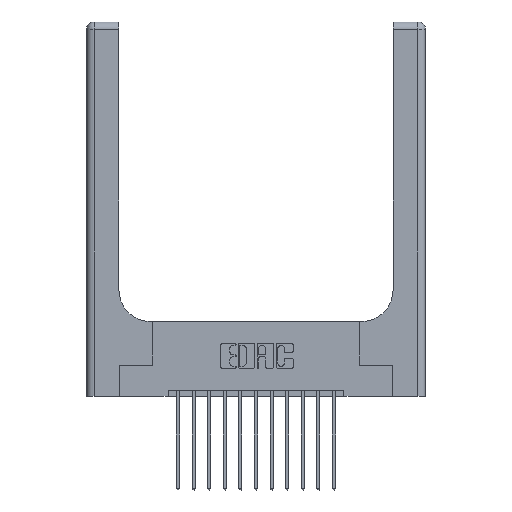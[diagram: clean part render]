
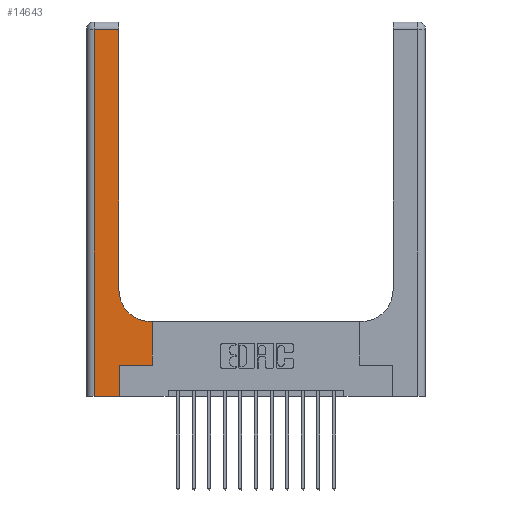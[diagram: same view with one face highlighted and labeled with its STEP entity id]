
A CAD part, top view. The second image highlights one B-rep face of the part: STEP entity #14643.
In plain terms, the highlighted planar face has unit normal (0, 0, 1).
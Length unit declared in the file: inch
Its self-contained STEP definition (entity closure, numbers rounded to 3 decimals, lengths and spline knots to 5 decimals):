
#331 = VERTEX_POINT ( 'NONE', #6728 ) ;
#406 = DIRECTION ( 'NONE',  ( 1., 0., 0. ) ) ;
#546 = AXIS2_PLACEMENT_3D ( 'NONE', #7891, #6509, #5565 ) ;
#683 = CARTESIAN_POINT ( 'NONE',  ( 0., 0., 0.37 ) ) ;
#867 = ORIENTED_EDGE ( 'NONE', *, *, #12381, .T. ) ;
#1134 = DIRECTION ( 'NONE',  ( 1., 0., 0. ) ) ;
#1318 = VECTOR ( 'NONE', #406, 39.37008 ) ;
#1915 = LINE ( 'NONE', #8308, #15357 ) ;
#1994 = CARTESIAN_POINT ( 'NONE',  ( 0.26, 3., 0.37 ) ) ;
#2024 = CARTESIAN_POINT ( 'NONE',  ( 0.265, 0., 0.37 ) ) ;
#2453 = EDGE_CURVE ( 'NONE', #5222, #16873, #16595, .T. ) ;
#2658 = ORIENTED_EDGE ( 'NONE', *, *, #14351, .T. ) ;
#2792 = LINE ( 'NONE', #9544, #14381 ) ;
#3600 = ORIENTED_EDGE ( 'NONE', *, *, #9124, .T. ) ;
#3899 = VECTOR ( 'NONE', #7274, 39.37008 ) ;
#4488 = EDGE_CURVE ( 'NONE', #12766, #331, #2792, .T. ) ;
#4630 = VERTEX_POINT ( 'NONE', #15559 ) ;
#4856 = LINE ( 'NONE', #13943, #6250 ) ;
#4868 = ORIENTED_EDGE ( 'NONE', *, *, #6604, .T. ) ;
#5110 = DIRECTION ( 'NONE',  ( 0., 0., -1. ) ) ;
#5222 = VERTEX_POINT ( 'NONE', #10909 ) ;
#5347 = CARTESIAN_POINT ( 'NONE',  ( 0., 2.94, 0.37 ) ) ;
#5565 = DIRECTION ( 'NONE',  ( -1., 0., 0. ) ) ;
#5965 = DIRECTION ( 'NONE',  ( 1., 0., 0. ) ) ;
#6250 = VECTOR ( 'NONE', #6973, 39.37008 ) ;
#6509 = DIRECTION ( 'NONE',  ( 0., 0., -1. ) ) ;
#6604 = EDGE_CURVE ( 'NONE', #9500, #4630, #4856, .T. ) ;
#6646 = LINE ( 'NONE', #5347, #14794 ) ;
#6728 = CARTESIAN_POINT ( 'NONE',  ( 0.51, 0.6, 0.37 ) ) ;
#6859 = VECTOR ( 'NONE', #13214, 39.37008 ) ;
#6973 = DIRECTION ( 'NONE',  ( 0., 1., 0. ) ) ;
#7111 = CARTESIAN_POINT ( 'NONE',  ( 0.06, 0., 0.37 ) ) ;
#7274 = DIRECTION ( 'NONE',  ( 0., 1., 0. ) ) ;
#7813 = PLANE ( 'NONE',  #546 ) ;
#7891 = CARTESIAN_POINT ( 'NONE',  ( 0., 3., 0.37 ) ) ;
#8070 = ORIENTED_EDGE ( 'NONE', *, *, #12610, .T. ) ;
#8198 = CARTESIAN_POINT ( 'NONE',  ( 0.528, 0.6, 0.37 ) ) ;
#8306 = ORIENTED_EDGE ( 'NONE', *, *, #2453, .T. ) ;
#8308 = CARTESIAN_POINT ( 'NONE',  ( 0.528, 0.25, 0.37 ) ) ;
#8700 = CARTESIAN_POINT ( 'NONE',  ( 0.06, 2.94, 0.37 ) ) ;
#9102 = VECTOR ( 'NONE', #5965, 39.37008 ) ;
#9120 = VERTEX_POINT ( 'NONE', #7111 ) ;
#9124 = EDGE_CURVE ( 'NONE', #14593, #12766, #1915, .T. ) ;
#9221 = EDGE_CURVE ( 'NONE', #16873, #15475, #6646, .T. ) ;
#9284 = FACE_OUTER_BOUND ( 'NONE', #14777, .T. ) ;
#9303 = EDGE_CURVE ( 'NONE', #9120, #9500, #13930, .T. ) ;
#9500 = VERTEX_POINT ( 'NONE', #2024 ) ;
#9507 = CARTESIAN_POINT ( 'NONE',  ( 0.26, 2.94, 0.37 ) ) ;
#9544 = CARTESIAN_POINT ( 'NONE',  ( 0.26, 0.6, 0.37 ) ) ;
#9590 = LINE ( 'NONE', #12201, #1318 ) ;
#9660 = CIRCLE ( 'NONE', #15935, 0.25 ) ;
#10626 = DIRECTION ( 'NONE',  ( -1., 0., 0. ) ) ;
#10909 = CARTESIAN_POINT ( 'NONE',  ( 0.26, 0.85, 0.37 ) ) ;
#11491 = CARTESIAN_POINT ( 'NONE',  ( 0.528, 0.25, 0.37 ) ) ;
#12176 = ORIENTED_EDGE ( 'NONE', *, *, #9303, .T. ) ;
#12201 = CARTESIAN_POINT ( 'NONE',  ( 0.265, 0.25, 0.37 ) ) ;
#12381 = EDGE_CURVE ( 'NONE', #4630, #14593, #9590, .T. ) ;
#12610 = EDGE_CURVE ( 'NONE', #15475, #9120, #15795, .T. ) ;
#12714 = DIRECTION ( 'NONE',  ( -1., 0., 0. ) ) ;
#12766 = VERTEX_POINT ( 'NONE', #8198 ) ;
#13214 = DIRECTION ( 'NONE',  ( 0., -1., 0. ) ) ;
#13377 = CARTESIAN_POINT ( 'NONE',  ( 0.06, 3., 0.37 ) ) ;
#13515 = ORIENTED_EDGE ( 'NONE', *, *, #4488, .T. ) ;
#13544 = DIRECTION ( 'NONE',  ( 0., 1., 0. ) ) ;
#13930 = LINE ( 'NONE', #683, #9102 ) ;
#13943 = CARTESIAN_POINT ( 'NONE',  ( 0.265, 0., 0.37 ) ) ;
#14351 = EDGE_CURVE ( 'NONE', #331, #5222, #9660, .T. ) ;
#14381 = VECTOR ( 'NONE', #12714, 39.37008 ) ;
#14593 = VERTEX_POINT ( 'NONE', #11491 ) ;
#14643 = ADVANCED_FACE ( 'NONE', ( #9284 ), #7813, .F. ) ;
#14777 = EDGE_LOOP ( 'NONE', ( #8306, #16808, #8070, #12176, #4868, #867, #3600, #13515, #2658 ) ) ;
#14794 = VECTOR ( 'NONE', #10626, 39.37008 ) ;
#15357 = VECTOR ( 'NONE', #13544, 39.37008 ) ;
#15475 = VERTEX_POINT ( 'NONE', #8700 ) ;
#15559 = CARTESIAN_POINT ( 'NONE',  ( 0.265, 0.25, 0.37 ) ) ;
#15795 = LINE ( 'NONE', #13377, #6859 ) ;
#15935 = AXIS2_PLACEMENT_3D ( 'NONE', #16789, #5110, #1134 ) ;
#16595 = LINE ( 'NONE', #1994, #3899 ) ;
#16789 = CARTESIAN_POINT ( 'NONE',  ( 0.51, 0.85, 0.37 ) ) ;
#16808 = ORIENTED_EDGE ( 'NONE', *, *, #9221, .T. ) ;
#16873 = VERTEX_POINT ( 'NONE', #9507 ) ;
